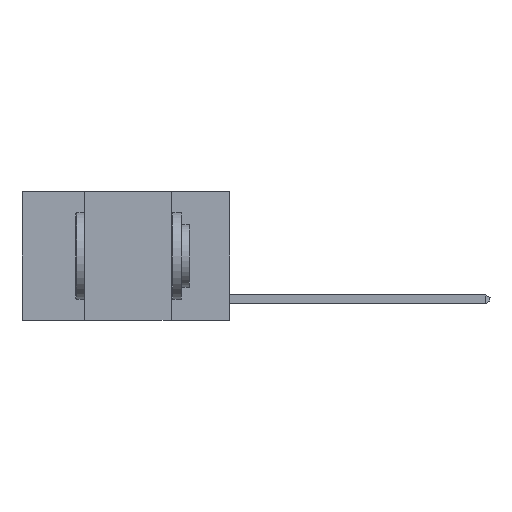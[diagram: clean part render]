
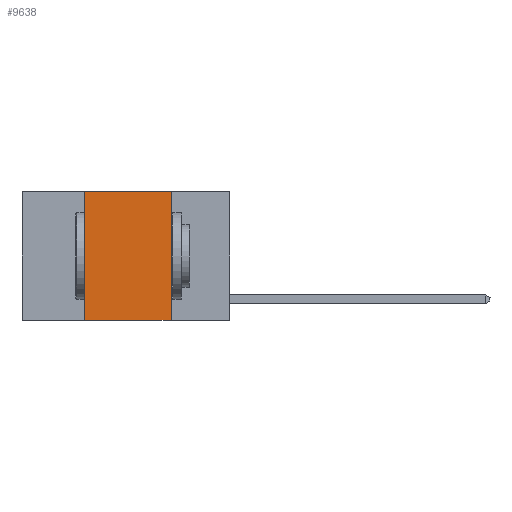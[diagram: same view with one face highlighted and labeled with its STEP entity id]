
A CAD part, left-side view. The second image highlights one B-rep face of the part: STEP entity #9638.
In plain terms, the highlighted planar face has unit normal (-1, 0, 0).
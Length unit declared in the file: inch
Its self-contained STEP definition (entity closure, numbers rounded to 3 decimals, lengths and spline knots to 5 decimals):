
#639 = VECTOR ( 'NONE', #13559, 39.37008 ) ;
#1515 = ORIENTED_EDGE ( 'NONE', *, *, #10136, .F. ) ;
#1864 = VECTOR ( 'NONE', #15837, 39.37008 ) ;
#3596 = LINE ( 'NONE', #18754, #11783 ) ;
#4653 = CARTESIAN_POINT ( 'NONE',  ( 0., 0.6, -0.37 ) ) ;
#4797 = FACE_OUTER_BOUND ( 'NONE', #5272, .T. ) ;
#5272 = EDGE_LOOP ( 'NONE', ( #17800, #1515, #15084, #8047 ) ) ;
#5336 = EDGE_CURVE ( 'NONE', #16055, #27728, #22579, .T. ) ;
#5715 = CARTESIAN_POINT ( 'NONE',  ( 0., 0.42, 0. ) ) ;
#6015 = CARTESIAN_POINT ( 'NONE',  ( 0., 0.42, -0.37 ) ) ;
#7870 = VERTEX_POINT ( 'NONE', #5715 ) ;
#8047 = ORIENTED_EDGE ( 'NONE', *, *, #5336, .T. ) ;
#8600 = PLANE ( 'NONE',  #21079 ) ;
#9142 = DIRECTION ( 'NONE',  ( 0., -1., 0. ) ) ;
#9638 = ADVANCED_FACE ( 'NONE', ( #4797 ), #8600, .F. ) ;
#10136 = EDGE_CURVE ( 'NONE', #7870, #23397, #11323, .T. ) ;
#11038 = LINE ( 'NONE', #26768, #1864 ) ;
#11323 = LINE ( 'NONE', #15839, #24093 ) ;
#11783 = VECTOR ( 'NONE', #28062, 39.37008 ) ;
#13559 = DIRECTION ( 'NONE',  ( 0., -1., 0. ) ) ;
#14085 = EDGE_CURVE ( 'NONE', #16055, #7870, #11038, .T. ) ;
#14876 = CARTESIAN_POINT ( 'NONE',  ( 0., 0.17, -0.37 ) ) ;
#15084 = ORIENTED_EDGE ( 'NONE', *, *, #14085, .F. ) ;
#15300 = DIRECTION ( 'NONE',  ( 1., 0., 0. ) ) ;
#15837 = DIRECTION ( 'NONE',  ( 0., 0., 1. ) ) ;
#15839 = CARTESIAN_POINT ( 'NONE',  ( 0., 0.6, 0. ) ) ;
#15872 = CARTESIAN_POINT ( 'NONE',  ( 0., 0.6, 0. ) ) ;
#16055 = VERTEX_POINT ( 'NONE', #6015 ) ;
#17800 = ORIENTED_EDGE ( 'NONE', *, *, #17953, .F. ) ;
#17953 = EDGE_CURVE ( 'NONE', #23397, #27728, #3596, .T. ) ;
#18754 = CARTESIAN_POINT ( 'NONE',  ( 0., 0.17, 0. ) ) ;
#19801 = DIRECTION ( 'NONE',  ( 0., 0., -1. ) ) ;
#21079 = AXIS2_PLACEMENT_3D ( 'NONE', #15872, #15300, #19801 ) ;
#22579 = LINE ( 'NONE', #4653, #639 ) ;
#23108 = CARTESIAN_POINT ( 'NONE',  ( 0., 0.17, 0. ) ) ;
#23397 = VERTEX_POINT ( 'NONE', #23108 ) ;
#24093 = VECTOR ( 'NONE', #9142, 39.37008 ) ;
#26768 = CARTESIAN_POINT ( 'NONE',  ( 0., 0.42, 0. ) ) ;
#27728 = VERTEX_POINT ( 'NONE', #14876 ) ;
#28062 = DIRECTION ( 'NONE',  ( 0., 0., -1. ) ) ;
